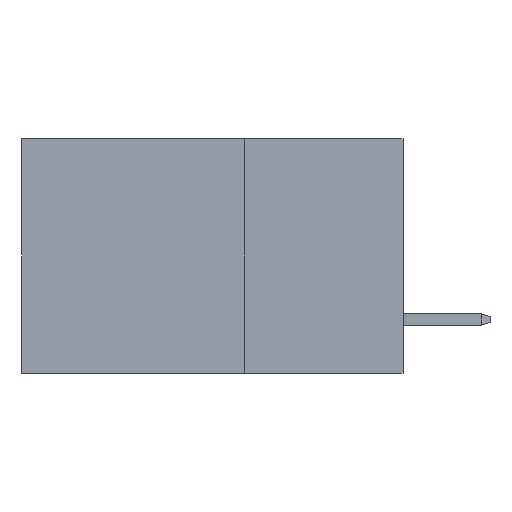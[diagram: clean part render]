
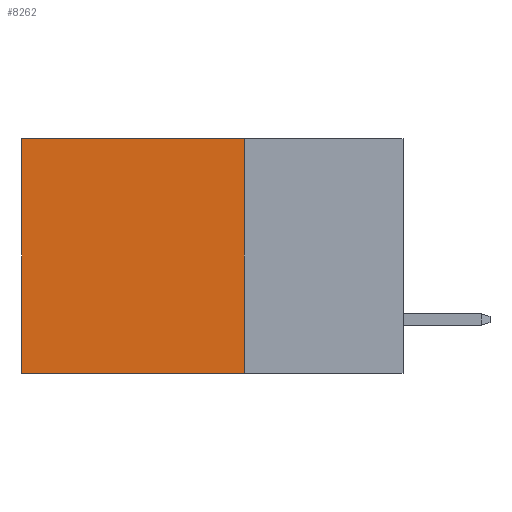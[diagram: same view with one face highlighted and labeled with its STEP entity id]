
A CAD part, left-side view. The second image highlights one B-rep face of the part: STEP entity #8262.
In plain terms, the highlighted planar face has unit normal (-1, 0, 0).
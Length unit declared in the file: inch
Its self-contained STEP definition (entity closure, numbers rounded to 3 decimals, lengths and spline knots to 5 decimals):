
#165 = ORIENTED_EDGE ( 'NONE', *, *, #7891, .T. ) ;
#316 = EDGE_CURVE ( 'NONE', #3865, #7933, #5698, .T. ) ;
#394 = CARTESIAN_POINT ( 'NONE',  ( 0.2875, 0.6, 0. ) ) ;
#1251 = CARTESIAN_POINT ( 'NONE',  ( 0.2875, 0.6, 0. ) ) ;
#1426 = CARTESIAN_POINT ( 'NONE',  ( 0.2875, 0.25, 0. ) ) ;
#1464 = CARTESIAN_POINT ( 'NONE',  ( 0.2875, 0.25, 0. ) ) ;
#1563 = ORIENTED_EDGE ( 'NONE', *, *, #6340, .F. ) ;
#2511 = VERTEX_POINT ( 'NONE', #394 ) ;
#2918 = DIRECTION ( 'NONE',  ( 0., 0., -1. ) ) ;
#3050 = AXIS2_PLACEMENT_3D ( 'NONE', #7798, #10329, #2918 ) ;
#3201 = CARTESIAN_POINT ( 'NONE',  ( 0.2875, 0.6, -0.37 ) ) ;
#3625 = CARTESIAN_POINT ( 'NONE',  ( 0.2875, 0.25, 0. ) ) ;
#3758 = LINE ( 'NONE', #1426, #5408 ) ;
#3798 = LINE ( 'NONE', #1464, #9602 ) ;
#3865 = VERTEX_POINT ( 'NONE', #6054 ) ;
#3878 = VERTEX_POINT ( 'NONE', #3625 ) ;
#4443 = DIRECTION ( 'NONE',  ( 0., 0., -1. ) ) ;
#4511 = PLANE ( 'NONE',  #3050 ) ;
#5039 = DIRECTION ( 'NONE',  ( 0., 1., 0. ) ) ;
#5144 = VECTOR ( 'NONE', #5039, 39.37008 ) ;
#5408 = VECTOR ( 'NONE', #8054, 39.37008 ) ;
#5698 = LINE ( 'NONE', #7337, #5144 ) ;
#6054 = CARTESIAN_POINT ( 'NONE',  ( 0.2875, 0.25, -0.37 ) ) ;
#6340 = EDGE_CURVE ( 'NONE', #3878, #3865, #3758, .T. ) ;
#6435 = DIRECTION ( 'NONE',  ( 0., 1., 0. ) ) ;
#6515 = VECTOR ( 'NONE', #4443, 39.37008 ) ;
#6548 = ORIENTED_EDGE ( 'NONE', *, *, #9083, .T. ) ;
#7337 = CARTESIAN_POINT ( 'NONE',  ( 0.2875, 0.25, -0.37 ) ) ;
#7798 = CARTESIAN_POINT ( 'NONE',  ( 0.2875, 0.25, 0. ) ) ;
#7891 = EDGE_CURVE ( 'NONE', #3878, #2511, #3798, .T. ) ;
#7933 = VERTEX_POINT ( 'NONE', #3201 ) ;
#8054 = DIRECTION ( 'NONE',  ( 0., 0., -1. ) ) ;
#8262 = ADVANCED_FACE ( 'NONE', ( #8646 ), #4511, .F. ) ;
#8646 = FACE_OUTER_BOUND ( 'NONE', #9855, .T. ) ;
#9083 = EDGE_CURVE ( 'NONE', #2511, #7933, #10359, .T. ) ;
#9501 = ORIENTED_EDGE ( 'NONE', *, *, #316, .F. ) ;
#9602 = VECTOR ( 'NONE', #6435, 39.37008 ) ;
#9855 = EDGE_LOOP ( 'NONE', ( #6548, #9501, #1563, #165 ) ) ;
#10329 = DIRECTION ( 'NONE',  ( 1., 0., 0. ) ) ;
#10359 = LINE ( 'NONE', #1251, #6515 ) ;
